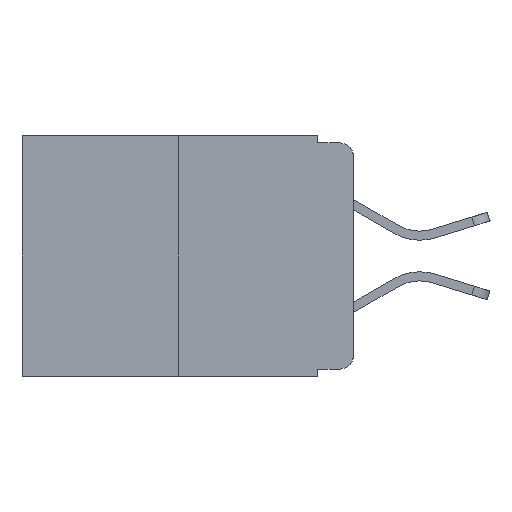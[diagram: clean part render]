
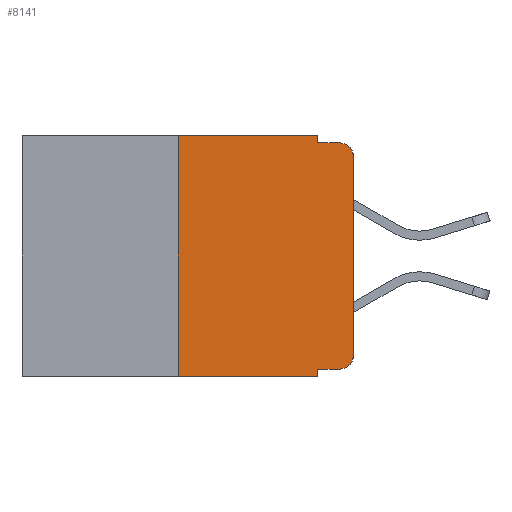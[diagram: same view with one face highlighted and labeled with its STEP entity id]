
A CAD part, left-side view. The second image highlights one B-rep face of the part: STEP entity #8141.
In plain terms, the highlighted planar face has unit normal (-1, 0, 0).
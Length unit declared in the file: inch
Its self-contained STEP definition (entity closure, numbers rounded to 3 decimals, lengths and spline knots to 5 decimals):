
#273 = EDGE_CURVE ( 'NONE', #9113, #3588, #1507, .T. ) ;
#781 = CARTESIAN_POINT ( 'NONE',  ( 0., 0.051, -0.333 ) ) ;
#1045 = ORIENTED_EDGE ( 'NONE', *, *, #6531, .F. ) ;
#1180 = PLANE ( 'NONE',  #8895 ) ;
#1190 = LINE ( 'NONE', #6662, #8264 ) ;
#1202 = CARTESIAN_POINT ( 'NONE',  ( 0., 0.25, 0. ) ) ;
#1316 = LINE ( 'NONE', #7570, #3535 ) ;
#1332 = ORIENTED_EDGE ( 'NONE', *, *, #7446, .F. ) ;
#1371 = AXIS2_PLACEMENT_3D ( 'NONE', #2113, #8537, #3067 ) ;
#1423 = CARTESIAN_POINT ( 'NONE',  ( 0., 0.02, -0.03 ) ) ;
#1507 = LINE ( 'NONE', #8115, #8595 ) ;
#2113 = CARTESIAN_POINT ( 'NONE',  ( 0., 0.02, -0.313 ) ) ;
#2219 = ORIENTED_EDGE ( 'NONE', *, *, #9690, .T. ) ;
#2241 = CARTESIAN_POINT ( 'NONE',  ( 0., 0.051, 0. ) ) ;
#2397 = DIRECTION ( 'NONE',  ( 0., 0., -1. ) ) ;
#2510 = VERTEX_POINT ( 'NONE', #5423 ) ;
#2534 = VECTOR ( 'NONE', #9017, 39.37008 ) ;
#2578 = CARTESIAN_POINT ( 'NONE',  ( 0., 0., -0.313 ) ) ;
#2584 = FACE_OUTER_BOUND ( 'NONE', #3669, .T. ) ;
#2613 = VERTEX_POINT ( 'NONE', #8461 ) ;
#2717 = AXIS2_PLACEMENT_3D ( 'NONE', #1423, #7931, #2397 ) ;
#3067 = DIRECTION ( 'NONE',  ( 0., 0., -1. ) ) ;
#3090 = DIRECTION ( 'NONE',  ( 0., 0., -1. ) ) ;
#3173 = CIRCLE ( 'NONE', #2717, 0.02 ) ;
#3262 = ORIENTED_EDGE ( 'NONE', *, *, #8903, .T. ) ;
#3356 = CARTESIAN_POINT ( 'NONE',  ( 0., 0.473, 0. ) ) ;
#3535 = VECTOR ( 'NONE', #4835, 39.37008 ) ;
#3556 = ORIENTED_EDGE ( 'NONE', *, *, #5946, .F. ) ;
#3588 = VERTEX_POINT ( 'NONE', #8291 ) ;
#3669 = EDGE_LOOP ( 'NONE', ( #7860, #3262, #1045, #3556, #1332, #3877, #8687, #6588, #11152, #2219 ) ) ;
#3877 = ORIENTED_EDGE ( 'NONE', *, *, #4709, .F. ) ;
#4211 = VERTEX_POINT ( 'NONE', #10695 ) ;
#4274 = VECTOR ( 'NONE', #5784, 39.37008 ) ;
#4311 = DIRECTION ( 'NONE',  ( 0., -1., 0. ) ) ;
#4709 = EDGE_CURVE ( 'NONE', #6460, #2510, #9203, .T. ) ;
#4737 = CARTESIAN_POINT ( 'NONE',  ( 0., 0.25, -0.343 ) ) ;
#4835 = DIRECTION ( 'NONE',  ( 0., 0., -1. ) ) ;
#5423 = CARTESIAN_POINT ( 'NONE',  ( 0., 0.25, 0. ) ) ;
#5694 = CARTESIAN_POINT ( 'NONE',  ( 0., 0.051, -0.01 ) ) ;
#5784 = DIRECTION ( 'NONE',  ( 0., -1., 0. ) ) ;
#5946 = EDGE_CURVE ( 'NONE', #6747, #4211, #1316, .T. ) ;
#6460 = VERTEX_POINT ( 'NONE', #4737 ) ;
#6531 = EDGE_CURVE ( 'NONE', #4211, #8325, #9030, .T. ) ;
#6588 = ORIENTED_EDGE ( 'NONE', *, *, #273, .F. ) ;
#6647 = VERTEX_POINT ( 'NONE', #9424 ) ;
#6662 = CARTESIAN_POINT ( 'NONE',  ( 0., 0.051, -0.333 ) ) ;
#6747 = VERTEX_POINT ( 'NONE', #2241 ) ;
#6881 = VECTOR ( 'NONE', #10929, 39.37008 ) ;
#7046 = CARTESIAN_POINT ( 'NONE',  ( 0., 0.02, -0.01 ) ) ;
#7230 = DIRECTION ( 'NONE',  ( 0., -1., 0. ) ) ;
#7446 = EDGE_CURVE ( 'NONE', #2510, #6747, #8216, .T. ) ;
#7570 = CARTESIAN_POINT ( 'NONE',  ( 0., 0.051, 0. ) ) ;
#7575 = DIRECTION ( 'NONE',  ( 0., -1., 0. ) ) ;
#7678 = CARTESIAN_POINT ( 'NONE',  ( 0., 0.473, 0. ) ) ;
#7860 = ORIENTED_EDGE ( 'NONE', *, *, #10573, .T. ) ;
#7931 = DIRECTION ( 'NONE',  ( -1., 0., 0. ) ) ;
#7945 = VECTOR ( 'NONE', #4311, 39.37008 ) ;
#8115 = CARTESIAN_POINT ( 'NONE',  ( 0., 0.051, 0. ) ) ;
#8141 = ADVANCED_FACE ( 'NONE', ( #2584 ), #1180, .F. ) ;
#8173 = CARTESIAN_POINT ( 'NONE',  ( 0., 0., 0. ) ) ;
#8216 = LINE ( 'NONE', #3356, #7945 ) ;
#8264 = VECTOR ( 'NONE', #7575, 39.37008 ) ;
#8291 = CARTESIAN_POINT ( 'NONE',  ( 0., 0.051, -0.343 ) ) ;
#8325 = VERTEX_POINT ( 'NONE', #7046 ) ;
#8442 = VECTOR ( 'NONE', #7230, 39.37008 ) ;
#8461 = CARTESIAN_POINT ( 'NONE',  ( 0., 0., -0.03 ) ) ;
#8537 = DIRECTION ( 'NONE',  ( -1., 0., 0. ) ) ;
#8562 = DIRECTION ( 'NONE',  ( 1., 0., 0. ) ) ;
#8595 = VECTOR ( 'NONE', #9580, 39.37008 ) ;
#8687 = ORIENTED_EDGE ( 'NONE', *, *, #9046, .T. ) ;
#8895 = AXIS2_PLACEMENT_3D ( 'NONE', #7678, #8562, #3090 ) ;
#8903 = EDGE_CURVE ( 'NONE', #2613, #8325, #3173, .T. ) ;
#9017 = DIRECTION ( 'NONE',  ( 0., 0., 1. ) ) ;
#9030 = LINE ( 'NONE', #5694, #4274 ) ;
#9046 = EDGE_CURVE ( 'NONE', #6460, #3588, #10941, .T. ) ;
#9113 = VERTEX_POINT ( 'NONE', #781 ) ;
#9203 = LINE ( 'NONE', #1202, #6881 ) ;
#9424 = CARTESIAN_POINT ( 'NONE',  ( 0., 0.02, -0.333 ) ) ;
#9580 = DIRECTION ( 'NONE',  ( 0., 0., -1. ) ) ;
#9690 = EDGE_CURVE ( 'NONE', #6647, #10552, #10786, .T. ) ;
#9751 = LINE ( 'NONE', #8173, #2534 ) ;
#10552 = VERTEX_POINT ( 'NONE', #2578 ) ;
#10573 = EDGE_CURVE ( 'NONE', #10552, #2613, #9751, .T. ) ;
#10695 = CARTESIAN_POINT ( 'NONE',  ( 0., 0.051, -0.01 ) ) ;
#10786 = CIRCLE ( 'NONE', #1371, 0.02 ) ;
#10929 = DIRECTION ( 'NONE',  ( 0., 0., 1. ) ) ;
#10941 = LINE ( 'NONE', #11414, #8442 ) ;
#11152 = ORIENTED_EDGE ( 'NONE', *, *, #11325, .T. ) ;
#11325 = EDGE_CURVE ( 'NONE', #9113, #6647, #1190, .T. ) ;
#11414 = CARTESIAN_POINT ( 'NONE',  ( 0., 0.473, -0.343 ) ) ;
